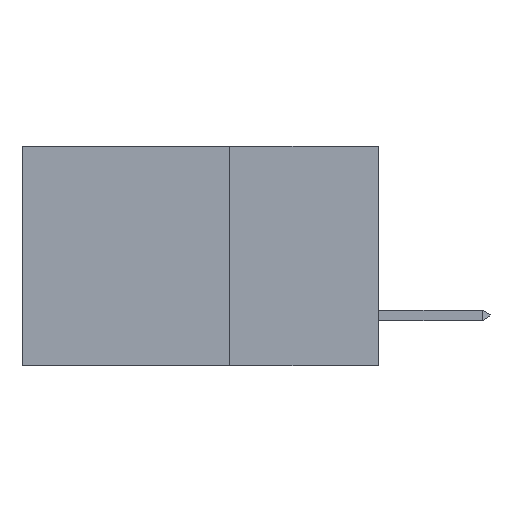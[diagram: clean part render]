
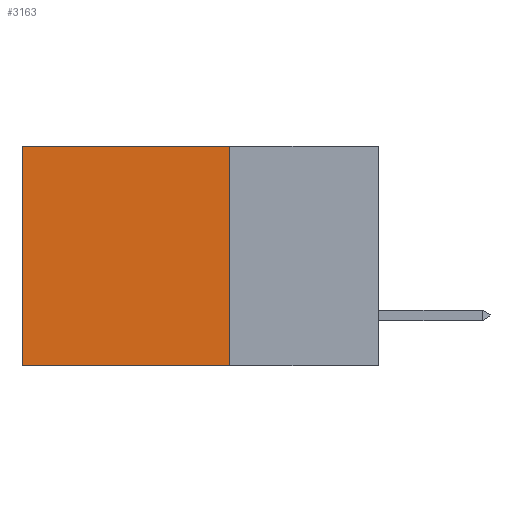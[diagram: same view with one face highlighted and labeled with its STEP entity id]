
A CAD part, left-side view. The second image highlights one B-rep face of the part: STEP entity #3163.
In plain terms, the highlighted planar face has unit normal (-1, 0, 0).
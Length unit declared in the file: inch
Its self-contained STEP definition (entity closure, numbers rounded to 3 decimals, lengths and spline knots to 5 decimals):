
#305 = FACE_OUTER_BOUND ( 'NONE', #13894, .T. ) ;
#469 = LINE ( 'NONE', #9738, #1177 ) ;
#770 = EDGE_CURVE ( 'NONE', #10213, #4441, #8437, .T. ) ;
#896 = DIRECTION ( 'NONE',  ( 0., 1., 0. ) ) ;
#1003 = CARTESIAN_POINT ( 'NONE',  ( 0.298, 0.25, -0.37 ) ) ;
#1146 = DIRECTION ( 'NONE',  ( 0., 0., -1. ) ) ;
#1177 = VECTOR ( 'NONE', #12120, 39.37008 ) ;
#1264 = VERTEX_POINT ( 'NONE', #3239 ) ;
#1939 = CARTESIAN_POINT ( 'NONE',  ( 0.298, 0.6, 0. ) ) ;
#2207 = AXIS2_PLACEMENT_3D ( 'NONE', #6393, #8576, #10781 ) ;
#2268 = VECTOR ( 'NONE', #14196, 39.37008 ) ;
#2355 = EDGE_CURVE ( 'NONE', #1264, #6065, #10804, .T. ) ;
#3163 = ADVANCED_FACE ( 'NONE', ( #305 ), #5194, .F. ) ;
#3239 = CARTESIAN_POINT ( 'NONE',  ( 0.298, 0.25, 0. ) ) ;
#4139 = VECTOR ( 'NONE', #896, 39.37008 ) ;
#4441 = VERTEX_POINT ( 'NONE', #7139 ) ;
#4653 = CARTESIAN_POINT ( 'NONE',  ( 0.298, 0.6, 0. ) ) ;
#5194 = PLANE ( 'NONE',  #2207 ) ;
#6065 = VERTEX_POINT ( 'NONE', #1003 ) ;
#6210 = CARTESIAN_POINT ( 'NONE',  ( 0.298, 0.25, 0. ) ) ;
#6393 = CARTESIAN_POINT ( 'NONE',  ( 0.298, 0.25, 0. ) ) ;
#6541 = CARTESIAN_POINT ( 'NONE',  ( 0.298, 0.25, 0. ) ) ;
#7139 = CARTESIAN_POINT ( 'NONE',  ( 0.298, 0.6, -0.37 ) ) ;
#7620 = ORIENTED_EDGE ( 'NONE', *, *, #770, .T. ) ;
#8020 = EDGE_CURVE ( 'NONE', #6065, #4441, #469, .T. ) ;
#8437 = LINE ( 'NONE', #4653, #9875 ) ;
#8576 = DIRECTION ( 'NONE',  ( 1., 0., 0. ) ) ;
#9738 = CARTESIAN_POINT ( 'NONE',  ( 0.298, 0.25, -0.37 ) ) ;
#9875 = VECTOR ( 'NONE', #1146, 39.37008 ) ;
#9877 = EDGE_CURVE ( 'NONE', #1264, #10213, #13202, .T. ) ;
#10213 = VERTEX_POINT ( 'NONE', #1939 ) ;
#10781 = DIRECTION ( 'NONE',  ( 0., 0., -1. ) ) ;
#10804 = LINE ( 'NONE', #6210, #2268 ) ;
#11884 = ORIENTED_EDGE ( 'NONE', *, *, #9877, .T. ) ;
#12120 = DIRECTION ( 'NONE',  ( 0., 1., 0. ) ) ;
#13202 = LINE ( 'NONE', #6541, #4139 ) ;
#13859 = ORIENTED_EDGE ( 'NONE', *, *, #2355, .F. ) ;
#13894 = EDGE_LOOP ( 'NONE', ( #7620, #13957, #13859, #11884 ) ) ;
#13957 = ORIENTED_EDGE ( 'NONE', *, *, #8020, .F. ) ;
#14196 = DIRECTION ( 'NONE',  ( 0., 0., -1. ) ) ;
